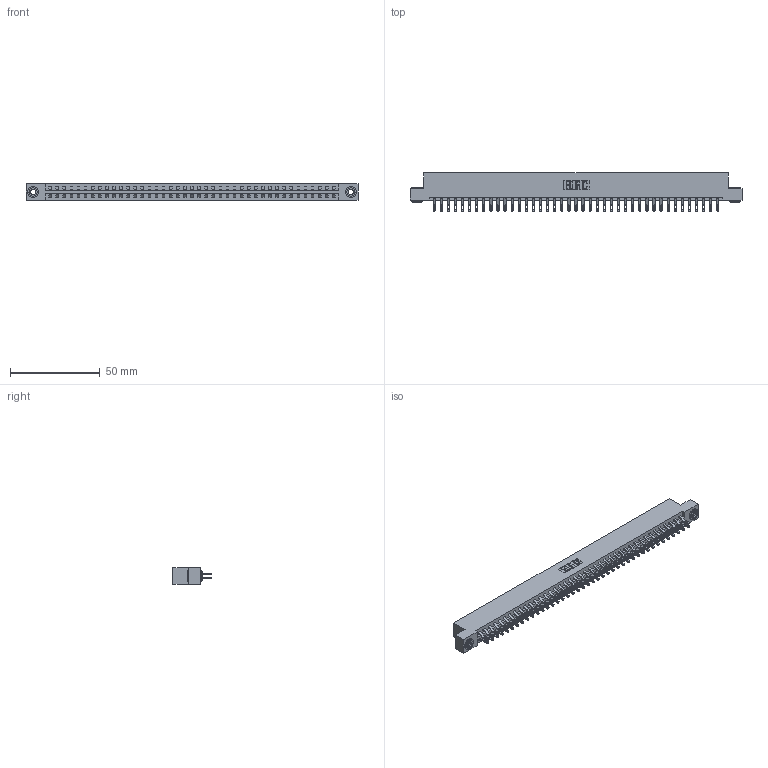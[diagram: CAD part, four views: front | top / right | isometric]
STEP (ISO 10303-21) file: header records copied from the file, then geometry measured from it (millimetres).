
FILE_DESCRIPTION (( 'STEP AP203' ), '1' );
FILE_NAME ('387-082-555-203.STEP', '2019-10-23T00:05:23', ( '' ), ( '' ), 'SwSTEP 2.0', 'SolidWorks 2016', '' );
FILE_SCHEMA (( 'CONFIG_CONTROL_DESIGN' ));
Length unit declared in the file: inch
Products named in the file (4): 345-250-002_345-250-002-102; 387-082-555-203; 337 Part_Flush Mounting Lugs - 0.156 Dia-TH; 345-292-001_555 Tail
Assembly tree (85 placements, depth 2):
  387-082-555-203
    337 Part_Flush Mounting Lugs - 0.156 Dia-TH
    345-292-001_555 Tail  x82
    345-250-002_345-250-002-102  x2
Bounding box: 185.47 x 21.47 x 9.4 mm (x, y, z)
Volume: 19790.3 mm3; surface area: 23484 mm2
Topology: 85 solids, 85 shells, 5072 faces, 15885 edges, 10586 vertices
Faces by surface type: plane 3032, cylinder 2032, cone 8
Entity records: 32894 total; most frequent: CARTESIAN_POINT 5551, ORIENTED_EDGE 5450, DIRECTION 4727, EDGE_CURVE 2725, VECTOR 2553, LINE 2553, VERTEX_POINT 1814, AXIS2_PLACEMENT_3D 1087
